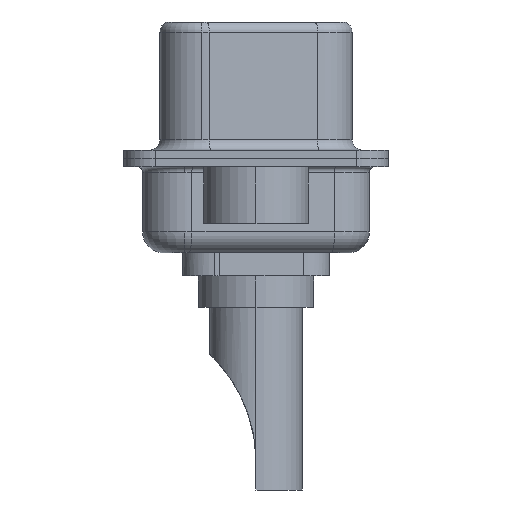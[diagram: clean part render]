
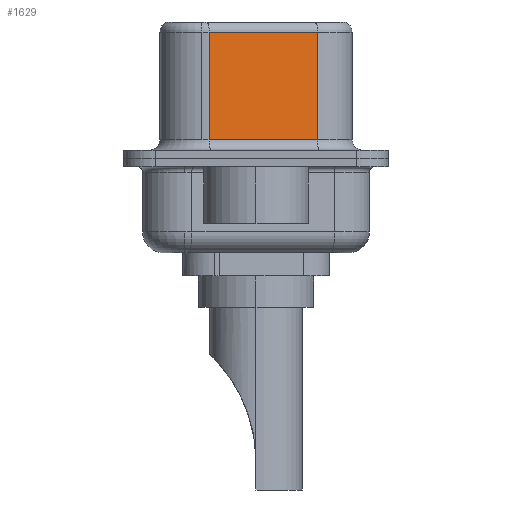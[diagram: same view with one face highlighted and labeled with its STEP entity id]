
A CAD part, left-side view. The second image highlights one B-rep face of the part: STEP entity #1629.
In plain terms, the highlighted planar face has unit normal (-0.985, -0.174, 0).
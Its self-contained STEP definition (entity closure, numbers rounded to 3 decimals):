
#854 = ORIENTED_EDGE ( 'NONE', *, *, #7344, .F. ) ;
#1155 = ORIENTED_EDGE ( 'NONE', *, *, #7363, .T. ) ;
#1629 = ADVANCED_FACE ( 'NONE', ( #14388 ), #9364, .F. ) ;
#1712 = CARTESIAN_POINT ( 'NONE',  ( 4.585, -2.927, 0.9 ) ) ;
#3082 = DIRECTION ( 'NONE',  ( 0.174, -0.985, 0. ) ) ;
#3422 = AXIS2_PLACEMENT_3D ( 'NONE', #9923, #9086, #8843 ) ;
#3474 = LINE ( 'NONE', #4141, #17150 ) ;
#3924 = VECTOR ( 'NONE', #8125, 1000. ) ;
#4141 = CARTESIAN_POINT ( 'NONE',  ( 3.675, 2.233, 6.52 ) ) ;
#4908 = DIRECTION ( 'NONE',  ( -0.174, 0.985, 0. ) ) ;
#5286 = LINE ( 'NONE', #1712, #14868 ) ;
#5901 = ORIENTED_EDGE ( 'NONE', *, *, #9602, .T. ) ;
#6802 = CARTESIAN_POINT ( 'NONE',  ( 4.585, -2.927, 6.52 ) ) ;
#6941 = VECTOR ( 'NONE', #4908, 1000. ) ;
#7304 = VERTEX_POINT ( 'NONE', #8073 ) ;
#7344 = EDGE_CURVE ( 'NONE', #7304, #13232, #7826, .T. ) ;
#7363 = EDGE_CURVE ( 'NONE', #9336, #12710, #3474, .T. ) ;
#7826 = LINE ( 'NONE', #6802, #3924 ) ;
#8073 = CARTESIAN_POINT ( 'NONE',  ( 4.585, -2.927, 6.02 ) ) ;
#8125 = DIRECTION ( 'NONE',  ( 0., 0., -1. ) ) ;
#8229 = ORIENTED_EDGE ( 'NONE', *, *, #10875, .T. ) ;
#8843 = DIRECTION ( 'NONE',  ( -0.174, 0.985, 0. ) ) ;
#9086 = DIRECTION ( 'NONE',  ( 0.985, 0.174, 0. ) ) ;
#9209 = CARTESIAN_POINT ( 'NONE',  ( 3.675, 2.233, 0.9 ) ) ;
#9336 = VERTEX_POINT ( 'NONE', #12330 ) ;
#9364 = PLANE ( 'NONE',  #3422 ) ;
#9602 = EDGE_CURVE ( 'NONE', #7304, #9336, #14335, .T. ) ;
#9712 = EDGE_LOOP ( 'NONE', ( #854, #5901, #1155, #8229 ) ) ;
#9923 = CARTESIAN_POINT ( 'NONE',  ( 4.585, -2.927, 6.52 ) ) ;
#10875 = EDGE_CURVE ( 'NONE', #12710, #13232, #5286, .T. ) ;
#11642 = CARTESIAN_POINT ( 'NONE',  ( 4.585, -2.927, 0.9 ) ) ;
#12095 = DIRECTION ( 'NONE',  ( 0., 0., -1. ) ) ;
#12330 = CARTESIAN_POINT ( 'NONE',  ( 3.675, 2.233, 6.02 ) ) ;
#12710 = VERTEX_POINT ( 'NONE', #9209 ) ;
#12782 = CARTESIAN_POINT ( 'NONE',  ( 4.585, -2.927, 6.02 ) ) ;
#13232 = VERTEX_POINT ( 'NONE', #11642 ) ;
#14335 = LINE ( 'NONE', #12782, #6941 ) ;
#14388 = FACE_OUTER_BOUND ( 'NONE', #9712, .T. ) ;
#14868 = VECTOR ( 'NONE', #3082, 1000. ) ;
#17150 = VECTOR ( 'NONE', #12095, 1000. ) ;
